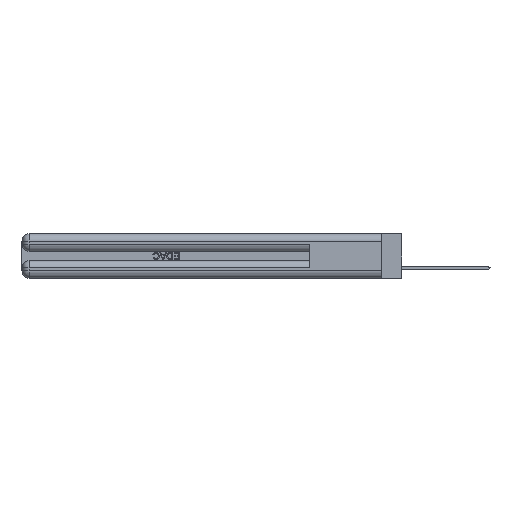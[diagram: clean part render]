
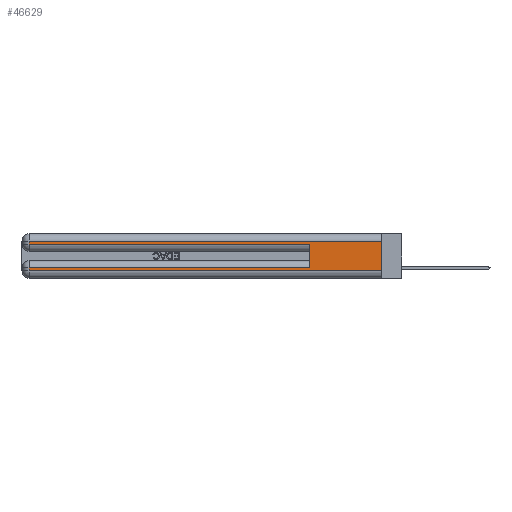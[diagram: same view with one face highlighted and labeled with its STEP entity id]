
A CAD part, left-side view. The second image highlights one B-rep face of the part: STEP entity #46629.
In plain terms, the highlighted planar face has unit normal (-1, 0, 0).
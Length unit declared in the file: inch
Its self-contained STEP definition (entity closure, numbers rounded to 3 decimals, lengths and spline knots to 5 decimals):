
#1257 = LINE ( 'NONE', #21617, #11350 ) ;
#2292 = VERTEX_POINT ( 'NONE', #49408 ) ;
#3202 = PLANE ( 'NONE',  #17022 ) ;
#3531 = DIRECTION ( 'NONE',  ( 0., 0., -1. ) ) ;
#3841 = DIRECTION ( 'NONE',  ( 0., 1., 0. ) ) ;
#5197 = VECTOR ( 'NONE', #51283, 39.37008 ) ;
#6688 = LINE ( 'NONE', #24372, #23238 ) ;
#7937 = ORIENTED_EDGE ( 'NONE', *, *, #31707, .T. ) ;
#8396 = CARTESIAN_POINT ( 'NONE',  ( 0., 0.6, 0.145 ) ) ;
#11350 = VECTOR ( 'NONE', #34746, 39.37008 ) ;
#11827 = CARTESIAN_POINT ( 'NONE',  ( 0., 0., 0.37 ) ) ;
#12600 = DIRECTION ( 'NONE',  ( 0., -1., 0. ) ) ;
#13278 = EDGE_CURVE ( 'NONE', #53135, #18056, #36289, .T. ) ;
#14153 = ORIENTED_EDGE ( 'NONE', *, *, #42783, .T. ) ;
#14674 = VECTOR ( 'NONE', #3841, 39.37008 ) ;
#17022 = AXIS2_PLACEMENT_3D ( 'NONE', #32814, #33171, #28891 ) ;
#18056 = VERTEX_POINT ( 'NONE', #45235 ) ;
#18994 = ORIENTED_EDGE ( 'NONE', *, *, #42069, .F. ) ;
#21617 = CARTESIAN_POINT ( 'NONE',  ( 0., 0., 0.06 ) ) ;
#22714 = VECTOR ( 'NONE', #12600, 39.37008 ) ;
#23238 = VECTOR ( 'NONE', #3531, 39.37008 ) ;
#24372 = CARTESIAN_POINT ( 'NONE',  ( 0., 2.94, 0.37 ) ) ;
#25049 = LINE ( 'NONE', #38529, #49739 ) ;
#25724 = FACE_OUTER_BOUND ( 'NONE', #55243, .T. ) ;
#27082 = ORIENTED_EDGE ( 'NONE', *, *, #48612, .T. ) ;
#27359 = LINE ( 'NONE', #29671, #14674 ) ;
#28379 = ORIENTED_EDGE ( 'NONE', *, *, #13278, .T. ) ;
#28440 = DIRECTION ( 'NONE',  ( 0., 1., 0. ) ) ;
#28479 = VERTEX_POINT ( 'NONE', #34661 ) ;
#28786 = VECTOR ( 'NONE', #45773, 39.37008 ) ;
#28891 = DIRECTION ( 'NONE',  ( 0., 0., -1. ) ) ;
#29671 = CARTESIAN_POINT ( 'NONE',  ( 0., 0., 0.085 ) ) ;
#29698 = ORIENTED_EDGE ( 'NONE', *, *, #49179, .T. ) ;
#31707 = EDGE_CURVE ( 'NONE', #18056, #2292, #25049, .T. ) ;
#31753 = CARTESIAN_POINT ( 'NONE',  ( 0., 0., 0.31 ) ) ;
#32299 = CARTESIAN_POINT ( 'NONE',  ( 0., 2.94, 0.085 ) ) ;
#32535 = CARTESIAN_POINT ( 'NONE',  ( 0., 0., 0.31 ) ) ;
#32814 = CARTESIAN_POINT ( 'NONE',  ( 0., 0., 0.37 ) ) ;
#33171 = DIRECTION ( 'NONE',  ( 1., 0., 0. ) ) ;
#34661 = CARTESIAN_POINT ( 'NONE',  ( 0., 2.94, 0.06 ) ) ;
#34746 = DIRECTION ( 'NONE',  ( 0., -1., 0. ) ) ;
#35034 = VERTEX_POINT ( 'NONE', #35753 ) ;
#35753 = CARTESIAN_POINT ( 'NONE',  ( 0., 0., 0.06 ) ) ;
#36289 = LINE ( 'NONE', #32535, #41735 ) ;
#36493 = ORIENTED_EDGE ( 'NONE', *, *, #52972, .F. ) ;
#38362 = CARTESIAN_POINT ( 'NONE',  ( 0., 0., 0.285 ) ) ;
#38529 = CARTESIAN_POINT ( 'NONE',  ( 0., 2.94, 0.37 ) ) ;
#39179 = EDGE_CURVE ( 'NONE', #42016, #28479, #6688, .T. ) ;
#39375 = LINE ( 'NONE', #11827, #28786 ) ;
#39855 = LINE ( 'NONE', #8396, #5197 ) ;
#40901 = VERTEX_POINT ( 'NONE', #49971 ) ;
#41735 = VECTOR ( 'NONE', #28440, 39.37008 ) ;
#42016 = VERTEX_POINT ( 'NONE', #32299 ) ;
#42069 = EDGE_CURVE ( 'NONE', #53135, #35034, #39375, .T. ) ;
#42373 = CARTESIAN_POINT ( 'NONE',  ( 0., 0.6, 0.085 ) ) ;
#42783 = EDGE_CURVE ( 'NONE', #28479, #35034, #1257, .T. ) ;
#43105 = DIRECTION ( 'NONE',  ( 0., 0., -1. ) ) ;
#43696 = VERTEX_POINT ( 'NONE', #42373 ) ;
#43987 = ORIENTED_EDGE ( 'NONE', *, *, #39179, .T. ) ;
#45235 = CARTESIAN_POINT ( 'NONE',  ( 0., 2.94, 0.31 ) ) ;
#45773 = DIRECTION ( 'NONE',  ( 0., 0., -1. ) ) ;
#46629 = ADVANCED_FACE ( 'NONE', ( #25724 ), #3202, .F. ) ;
#48612 = EDGE_CURVE ( 'NONE', #2292, #40901, #50903, .T. ) ;
#49179 = EDGE_CURVE ( 'NONE', #43696, #42016, #27359, .T. ) ;
#49408 = CARTESIAN_POINT ( 'NONE',  ( 0., 2.94, 0.285 ) ) ;
#49739 = VECTOR ( 'NONE', #43105, 39.37008 ) ;
#49971 = CARTESIAN_POINT ( 'NONE',  ( 0., 0.6, 0.285 ) ) ;
#50903 = LINE ( 'NONE', #38362, #22714 ) ;
#51283 = DIRECTION ( 'NONE',  ( 0., 0., 1. ) ) ;
#52972 = EDGE_CURVE ( 'NONE', #43696, #40901, #39855, .T. ) ;
#53135 = VERTEX_POINT ( 'NONE', #31753 ) ;
#55243 = EDGE_LOOP ( 'NONE', ( #18994, #28379, #7937, #27082, #36493, #29698, #43987, #14153 ) ) ;
